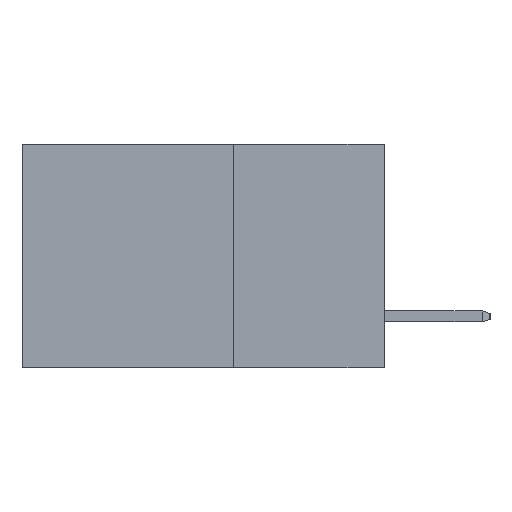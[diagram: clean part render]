
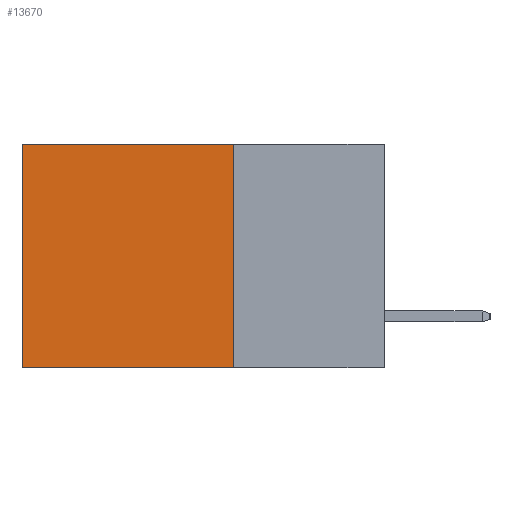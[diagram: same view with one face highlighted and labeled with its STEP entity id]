
A CAD part, left-side view. The second image highlights one B-rep face of the part: STEP entity #13670.
In plain terms, the highlighted planar face has unit normal (-1, 0, 0).
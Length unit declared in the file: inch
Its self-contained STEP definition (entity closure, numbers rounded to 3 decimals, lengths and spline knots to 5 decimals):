
#1594 = CARTESIAN_POINT ( 'NONE',  ( 0.2615, 0.25, -0.37 ) ) ;
#1991 = ORIENTED_EDGE ( 'NONE', *, *, #3773, .T. ) ;
#2460 = VERTEX_POINT ( 'NONE', #8666 ) ;
#2957 = VERTEX_POINT ( 'NONE', #9281 ) ;
#3403 = ORIENTED_EDGE ( 'NONE', *, *, #10359, .F. ) ;
#3647 = ORIENTED_EDGE ( 'NONE', *, *, #6629, .F. ) ;
#3725 = DIRECTION ( 'NONE',  ( 0., 0., -1. ) ) ;
#3766 = CARTESIAN_POINT ( 'NONE',  ( 0.2615, 0.6, -0.37 ) ) ;
#3773 = EDGE_CURVE ( 'NONE', #4119, #2460, #10070, .T. ) ;
#3897 = VERTEX_POINT ( 'NONE', #1594 ) ;
#4119 = VERTEX_POINT ( 'NONE', #10856 ) ;
#4178 = VECTOR ( 'NONE', #14220, 39.37008 ) ;
#4404 = LINE ( 'NONE', #11974, #7853 ) ;
#4844 = PLANE ( 'NONE',  #11869 ) ;
#4901 = DIRECTION ( 'NONE',  ( 1., 0., 0. ) ) ;
#4945 = LINE ( 'NONE', #6664, #4178 ) ;
#5959 = DIRECTION ( 'NONE',  ( 0., 0., -1. ) ) ;
#6629 = EDGE_CURVE ( 'NONE', #3897, #2460, #4404, .T. ) ;
#6664 = CARTESIAN_POINT ( 'NONE',  ( 0.2615, 0.25, 0. ) ) ;
#7853 = VECTOR ( 'NONE', #11554, 39.37008 ) ;
#8088 = VECTOR ( 'NONE', #5959, 39.37008 ) ;
#8666 = CARTESIAN_POINT ( 'NONE',  ( 0.2615, 0.6, -0.37 ) ) ;
#8819 = FACE_OUTER_BOUND ( 'NONE', #14557, .T. ) ;
#9281 = CARTESIAN_POINT ( 'NONE',  ( 0.2615, 0.25, 0. ) ) ;
#9713 = VECTOR ( 'NONE', #3725, 39.37008 ) ;
#10012 = LINE ( 'NONE', #10404, #8088 ) ;
#10070 = LINE ( 'NONE', #3766, #9713 ) ;
#10359 = EDGE_CURVE ( 'NONE', #2957, #3897, #10012, .T. ) ;
#10404 = CARTESIAN_POINT ( 'NONE',  ( 0.2615, 0.25, -0.37 ) ) ;
#10856 = CARTESIAN_POINT ( 'NONE',  ( 0.2615, 0.6, 0. ) ) ;
#11554 = DIRECTION ( 'NONE',  ( 0., 1., 0. ) ) ;
#11869 = AXIS2_PLACEMENT_3D ( 'NONE', #13672, #4901, #12675 ) ;
#11947 = EDGE_CURVE ( 'NONE', #2957, #4119, #4945, .T. ) ;
#11974 = CARTESIAN_POINT ( 'NONE',  ( 0.2615, 0.25, -0.37 ) ) ;
#12623 = ORIENTED_EDGE ( 'NONE', *, *, #11947, .T. ) ;
#12675 = DIRECTION ( 'NONE',  ( 0., 0., -1. ) ) ;
#13670 = ADVANCED_FACE ( 'NONE', ( #8819 ), #4844, .F. ) ;
#13672 = CARTESIAN_POINT ( 'NONE',  ( 0.2615, 0.25, -0.37 ) ) ;
#14220 = DIRECTION ( 'NONE',  ( 0., 1., 0. ) ) ;
#14557 = EDGE_LOOP ( 'NONE', ( #1991, #3647, #3403, #12623 ) ) ;
